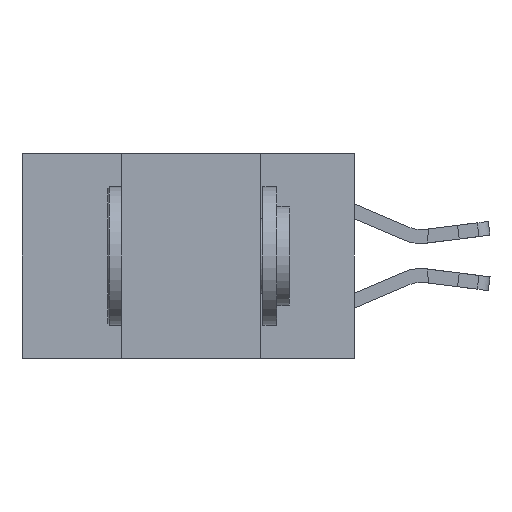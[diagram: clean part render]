
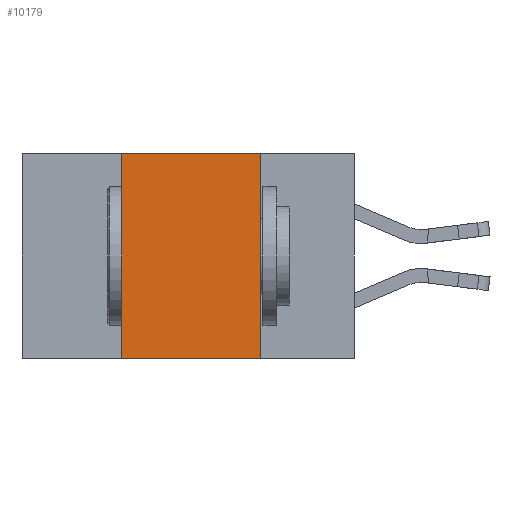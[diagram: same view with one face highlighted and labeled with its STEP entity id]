
A CAD part, left-side view. The second image highlights one B-rep face of the part: STEP entity #10179.
In plain terms, the highlighted planar face has unit normal (-1, 0, 0).
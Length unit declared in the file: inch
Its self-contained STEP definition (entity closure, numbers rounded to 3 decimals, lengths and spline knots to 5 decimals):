
#80 = EDGE_CURVE ( 'NONE', #5135, #11056, #4070, .T. ) ;
#108 = VECTOR ( 'NONE', #3650, 39.37008 ) ;
#621 = VECTOR ( 'NONE', #5708, 39.37008 ) ;
#887 = ORIENTED_EDGE ( 'NONE', *, *, #6021, .T. ) ;
#1627 = AXIS2_PLACEMENT_3D ( 'NONE', #8540, #8521, #8480 ) ;
#2247 = DIRECTION ( 'NONE',  ( 0., -1., 0. ) ) ;
#2435 = CARTESIAN_POINT ( 'NONE',  ( 0., 0.6, -0.37 ) ) ;
#3219 = DIRECTION ( 'NONE',  ( 0., 0., -1. ) ) ;
#3427 = VECTOR ( 'NONE', #2247, 39.37008 ) ;
#3571 = LINE ( 'NONE', #11297, #108 ) ;
#3650 = DIRECTION ( 'NONE',  ( 0., 0., 1. ) ) ;
#4070 = LINE ( 'NONE', #11851, #621 ) ;
#4903 = VECTOR ( 'NONE', #3219, 39.37008 ) ;
#5135 = VERTEX_POINT ( 'NONE', #13658 ) ;
#5708 = DIRECTION ( 'NONE',  ( 0., -1., 0. ) ) ;
#5883 = VERTEX_POINT ( 'NONE', #9361 ) ;
#6021 = EDGE_CURVE ( 'NONE', #11321, #5883, #13489, .T. ) ;
#7597 = CARTESIAN_POINT ( 'NONE',  ( 0., 0.42, -0.37 ) ) ;
#7974 = CARTESIAN_POINT ( 'NONE',  ( 0., 0.17, -0.37 ) ) ;
#8082 = ORIENTED_EDGE ( 'NONE', *, *, #80, .F. ) ;
#8287 = LINE ( 'NONE', #7974, #4903 ) ;
#8480 = DIRECTION ( 'NONE',  ( 0., 0., -1. ) ) ;
#8521 = DIRECTION ( 'NONE',  ( 1., 0., 0. ) ) ;
#8540 = CARTESIAN_POINT ( 'NONE',  ( 0., 0.6, 0. ) ) ;
#9337 = EDGE_LOOP ( 'NONE', ( #13178, #8082, #12415, #887 ) ) ;
#9361 = CARTESIAN_POINT ( 'NONE',  ( 0., 0.17, -0.37 ) ) ;
#10179 = ADVANCED_FACE ( 'NONE', ( #12012 ), #13438, .F. ) ;
#10215 = EDGE_CURVE ( 'NONE', #11056, #5883, #8287, .T. ) ;
#11056 = VERTEX_POINT ( 'NONE', #13303 ) ;
#11297 = CARTESIAN_POINT ( 'NONE',  ( 0., 0.42, -0.37 ) ) ;
#11321 = VERTEX_POINT ( 'NONE', #7597 ) ;
#11851 = CARTESIAN_POINT ( 'NONE',  ( 0., 0.6, 0. ) ) ;
#12012 = FACE_OUTER_BOUND ( 'NONE', #9337, .T. ) ;
#12415 = ORIENTED_EDGE ( 'NONE', *, *, #13242, .F. ) ;
#13178 = ORIENTED_EDGE ( 'NONE', *, *, #10215, .F. ) ;
#13242 = EDGE_CURVE ( 'NONE', #11321, #5135, #3571, .T. ) ;
#13303 = CARTESIAN_POINT ( 'NONE',  ( 0., 0.17, 0. ) ) ;
#13438 = PLANE ( 'NONE',  #1627 ) ;
#13489 = LINE ( 'NONE', #2435, #3427 ) ;
#13658 = CARTESIAN_POINT ( 'NONE',  ( 0., 0.42, 0. ) ) ;
